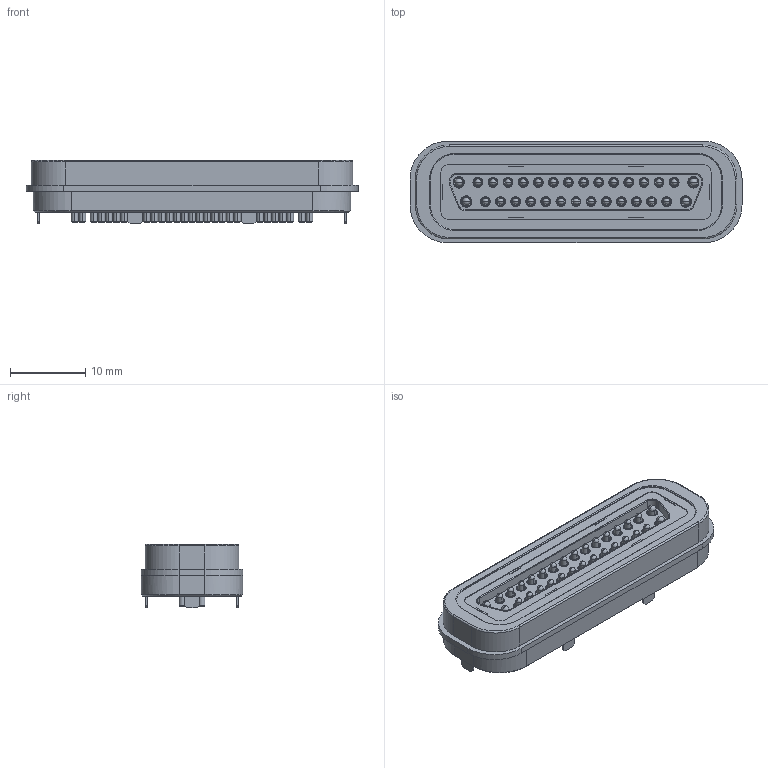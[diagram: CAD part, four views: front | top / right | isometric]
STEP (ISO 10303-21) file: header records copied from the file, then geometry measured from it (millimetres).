
FILE_DESCRIPTION (( 'STEP AP214' ), '1' );
FILE_NAME ('685A3131260111E.STEP', '2023-04-25T17:40:34', ( '' ), ( '' ), 'SwSTEP 2.0', 'SolidWorks 2020', '' );
FILE_SCHEMA (( 'AUTOMOTIVE_DESIGN' ));
Length unit declared in the file: millimetre
Products named in the file (1): 685A3131260111E
Bounding box: 43.98 x 13.44 x 8.35 mm (x, y, z)
Volume: 3102.3 mm3; surface area: 4778.9 mm2
Topology: 8 solids, 8 shells, 978 faces, 2274 edges, 1405 vertices
Faces by surface type: cylinder 386, plane 358, torus 88, cone 78, sphere 62, bspline 6
Entity records: 45315 total; most frequent: CARTESIAN_POINT 16863, ORIENTED_EDGE 4362, EDGE_CURVE 2181, DIRECTION 2110, B_SPLINE_CURVE_WITH_KNOTS 2039, VERTEX_POINT 1374, EDGE_LOOP 1143, AXIS2_PLACEMENT_3D 995
